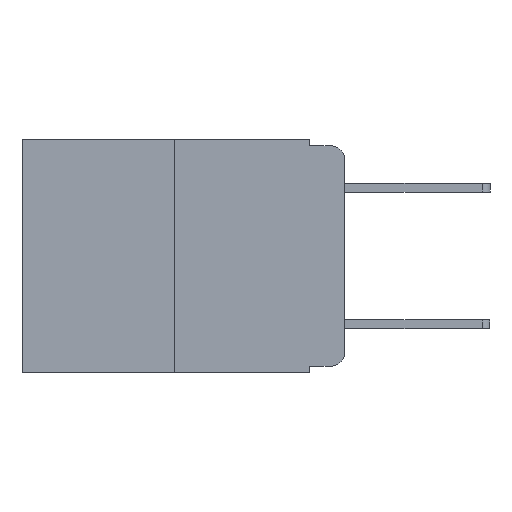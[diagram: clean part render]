
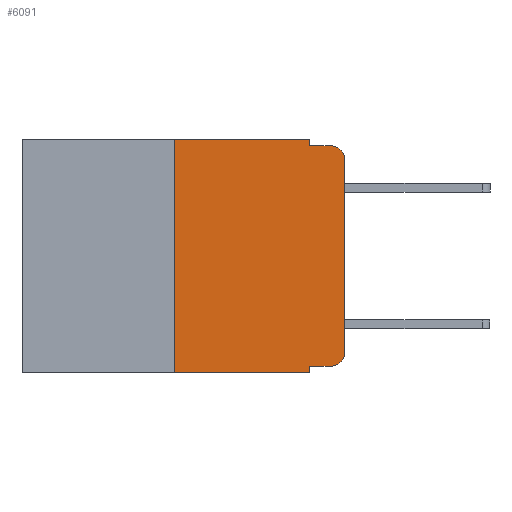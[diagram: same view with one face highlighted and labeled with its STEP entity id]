
A CAD part, left-side view. The second image highlights one B-rep face of the part: STEP entity #6091.
In plain terms, the highlighted planar face has unit normal (-1, 0, 0).
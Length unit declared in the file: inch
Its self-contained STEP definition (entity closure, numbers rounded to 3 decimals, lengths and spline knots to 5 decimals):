
#315 = LINE ( 'NONE', #11880, #15918 ) ;
#388 = ORIENTED_EDGE ( 'NONE', *, *, #9199, .T. ) ;
#503 = DIRECTION ( 'NONE',  ( 0., 0., 1. ) ) ;
#553 = DIRECTION ( 'NONE',  ( 0., 0., -1. ) ) ;
#588 = CARTESIAN_POINT ( 'NONE',  ( 0., 0.051, 0. ) ) ;
#1044 = DIRECTION ( 'NONE',  ( 0., 0., -1. ) ) ;
#1070 = EDGE_CURVE ( 'NONE', #11682, #14726, #315, .T. ) ;
#1155 = CARTESIAN_POINT ( 'NONE',  ( 0., 0.051, -0.333 ) ) ;
#1300 = DIRECTION ( 'NONE',  ( 0., -1., 0. ) ) ;
#1511 = CARTESIAN_POINT ( 'NONE',  ( 0., 0.473, 0. ) ) ;
#1601 = LINE ( 'NONE', #11418, #12877 ) ;
#1707 = CARTESIAN_POINT ( 'NONE',  ( 0., 0., -0.03 ) ) ;
#1790 = EDGE_CURVE ( 'NONE', #14726, #11078, #15221, .T. ) ;
#1883 = FACE_OUTER_BOUND ( 'NONE', #11178, .T. ) ;
#2147 = VERTEX_POINT ( 'NONE', #6554 ) ;
#2336 = VERTEX_POINT ( 'NONE', #1155 ) ;
#2668 = EDGE_CURVE ( 'NONE', #6059, #2147, #14614, .T. ) ;
#2892 = VECTOR ( 'NONE', #503, 39.37008 ) ;
#3200 = LINE ( 'NONE', #8856, #6644 ) ;
#3790 = CIRCLE ( 'NONE', #9683, 0.02 ) ;
#4455 = CARTESIAN_POINT ( 'NONE',  ( 0., 0.051, 0. ) ) ;
#4582 = CIRCLE ( 'NONE', #11183, 0.02 ) ;
#4702 = LINE ( 'NONE', #6017, #15884 ) ;
#5536 = DIRECTION ( 'NONE',  ( -1., 0., 0. ) ) ;
#5544 = EDGE_CURVE ( 'NONE', #2336, #6369, #4702, .T. ) ;
#5683 = CARTESIAN_POINT ( 'NONE',  ( 0., 0.051, -0.01 ) ) ;
#6017 = CARTESIAN_POINT ( 'NONE',  ( 0., 0.051, -0.333 ) ) ;
#6034 = DIRECTION ( 'NONE',  ( 0., -1., 0. ) ) ;
#6059 = VERTEX_POINT ( 'NONE', #17356 ) ;
#6091 = ADVANCED_FACE ( 'NONE', ( #1883 ), #14572, .F. ) ;
#6369 = VERTEX_POINT ( 'NONE', #12335 ) ;
#6540 = CARTESIAN_POINT ( 'NONE',  ( 0., 0., -0.313 ) ) ;
#6554 = CARTESIAN_POINT ( 'NONE',  ( 0., 0.25, 0. ) ) ;
#6644 = VECTOR ( 'NONE', #16168, 39.37008 ) ;
#6794 = EDGE_CURVE ( 'NONE', #2147, #11682, #16284, .T. ) ;
#6967 = LINE ( 'NONE', #588, #13855 ) ;
#7439 = VECTOR ( 'NONE', #1300, 39.37008 ) ;
#7940 = DIRECTION ( 'NONE',  ( 0., 0., -1. ) ) ;
#8776 = DIRECTION ( 'NONE',  ( 1., 0., 0. ) ) ;
#8856 = CARTESIAN_POINT ( 'NONE',  ( 0., 0., 0. ) ) ;
#8865 = CARTESIAN_POINT ( 'NONE',  ( 0., 0.051, -0.343 ) ) ;
#8894 = CARTESIAN_POINT ( 'NONE',  ( 0., 0.02, -0.01 ) ) ;
#9199 = EDGE_CURVE ( 'NONE', #6059, #15845, #1601, .T. ) ;
#9683 = AXIS2_PLACEMENT_3D ( 'NONE', #18571, #9853, #1044 ) ;
#9853 = DIRECTION ( 'NONE',  ( -1., 0., 0. ) ) ;
#9944 = DIRECTION ( 'NONE',  ( 0., -1., 0. ) ) ;
#10057 = ORIENTED_EDGE ( 'NONE', *, *, #5544, .T. ) ;
#10407 = EDGE_CURVE ( 'NONE', #16753, #11794, #3200, .T. ) ;
#10571 = AXIS2_PLACEMENT_3D ( 'NONE', #11635, #8776, #18919 ) ;
#11078 = VERTEX_POINT ( 'NONE', #8894 ) ;
#11178 = EDGE_LOOP ( 'NONE', ( #13026, #14399, #11891, #16667, #13733, #14637, #388, #16445, #10057, #14875 ) ) ;
#11183 = AXIS2_PLACEMENT_3D ( 'NONE', #14316, #5536, #15756 ) ;
#11418 = CARTESIAN_POINT ( 'NONE',  ( 0., 0.473, -0.343 ) ) ;
#11635 = CARTESIAN_POINT ( 'NONE',  ( 0., 0.473, 0. ) ) ;
#11682 = VERTEX_POINT ( 'NONE', #4455 ) ;
#11794 = VERTEX_POINT ( 'NONE', #1707 ) ;
#11880 = CARTESIAN_POINT ( 'NONE',  ( 0., 0.051, 0. ) ) ;
#11891 = ORIENTED_EDGE ( 'NONE', *, *, #1790, .F. ) ;
#12335 = CARTESIAN_POINT ( 'NONE',  ( 0., 0.02, -0.333 ) ) ;
#12429 = VECTOR ( 'NONE', #6034, 39.37008 ) ;
#12877 = VECTOR ( 'NONE', #9944, 39.37008 ) ;
#13026 = ORIENTED_EDGE ( 'NONE', *, *, #10407, .T. ) ;
#13733 = ORIENTED_EDGE ( 'NONE', *, *, #6794, .F. ) ;
#13855 = VECTOR ( 'NONE', #7940, 39.37008 ) ;
#14316 = CARTESIAN_POINT ( 'NONE',  ( 0., 0.02, -0.03 ) ) ;
#14399 = ORIENTED_EDGE ( 'NONE', *, *, #18807, .T. ) ;
#14572 = PLANE ( 'NONE',  #10571 ) ;
#14614 = LINE ( 'NONE', #18036, #2892 ) ;
#14637 = ORIENTED_EDGE ( 'NONE', *, *, #2668, .F. ) ;
#14726 = VERTEX_POINT ( 'NONE', #18591 ) ;
#14875 = ORIENTED_EDGE ( 'NONE', *, *, #15347, .T. ) ;
#15221 = LINE ( 'NONE', #5683, #7439 ) ;
#15347 = EDGE_CURVE ( 'NONE', #6369, #16753, #3790, .T. ) ;
#15756 = DIRECTION ( 'NONE',  ( 0., 0., -1. ) ) ;
#15845 = VERTEX_POINT ( 'NONE', #8865 ) ;
#15884 = VECTOR ( 'NONE', #17684, 39.37008 ) ;
#15918 = VECTOR ( 'NONE', #553, 39.37008 ) ;
#16073 = EDGE_CURVE ( 'NONE', #2336, #15845, #6967, .T. ) ;
#16168 = DIRECTION ( 'NONE',  ( 0., 0., 1. ) ) ;
#16284 = LINE ( 'NONE', #1511, #12429 ) ;
#16445 = ORIENTED_EDGE ( 'NONE', *, *, #16073, .F. ) ;
#16667 = ORIENTED_EDGE ( 'NONE', *, *, #1070, .F. ) ;
#16753 = VERTEX_POINT ( 'NONE', #6540 ) ;
#17356 = CARTESIAN_POINT ( 'NONE',  ( 0., 0.25, -0.343 ) ) ;
#17684 = DIRECTION ( 'NONE',  ( 0., -1., 0. ) ) ;
#18036 = CARTESIAN_POINT ( 'NONE',  ( 0., 0.25, 0. ) ) ;
#18571 = CARTESIAN_POINT ( 'NONE',  ( 0., 0.02, -0.313 ) ) ;
#18591 = CARTESIAN_POINT ( 'NONE',  ( 0., 0.051, -0.01 ) ) ;
#18807 = EDGE_CURVE ( 'NONE', #11794, #11078, #4582, .T. ) ;
#18919 = DIRECTION ( 'NONE',  ( 0., 0., -1. ) ) ;
